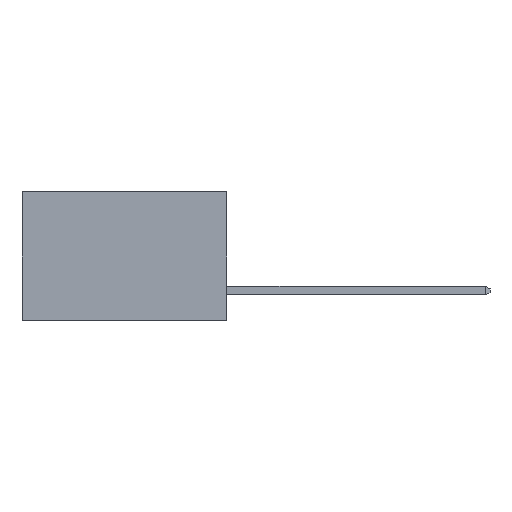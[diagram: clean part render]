
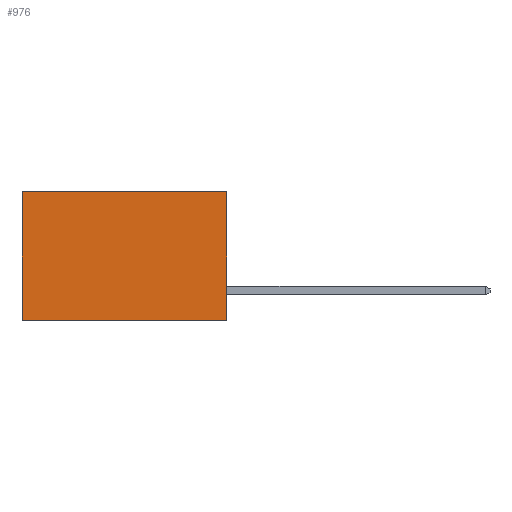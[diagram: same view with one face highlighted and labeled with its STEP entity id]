
A CAD part, left-side view. The second image highlights one B-rep face of the part: STEP entity #976.
In plain terms, the highlighted planar face has unit normal (-1, 0, 0).
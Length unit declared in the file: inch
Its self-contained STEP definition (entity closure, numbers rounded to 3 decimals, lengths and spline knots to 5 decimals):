
#465 = LINE ( 'NONE', #4557, #7526 ) ;
#525 = EDGE_CURVE ( 'NONE', #4774, #3673, #564, .T. ) ;
#564 = LINE ( 'NONE', #1978, #5940 ) ;
#807 = EDGE_CURVE ( 'NONE', #5442, #4774, #7591, .T. ) ;
#821 = CARTESIAN_POINT ( 'NONE',  ( 0.277, 0., -0.37 ) ) ;
#976 = ADVANCED_FACE ( 'NONE', ( #1510 ), #4227, .F. ) ;
#1510 = FACE_OUTER_BOUND ( 'NONE', #4595, .T. ) ;
#1978 = CARTESIAN_POINT ( 'NONE',  ( 0.277, 0., -0.37 ) ) ;
#2312 = DIRECTION ( 'NONE',  ( 0., 1., 0. ) ) ;
#2870 = AXIS2_PLACEMENT_3D ( 'NONE', #821, #4844, #5857 ) ;
#3120 = EDGE_CURVE ( 'NONE', #3223, #3673, #7224, .T. ) ;
#3223 = VERTEX_POINT ( 'NONE', #7795 ) ;
#3232 = CARTESIAN_POINT ( 'NONE',  ( 0.277, 0.59, -0.37 ) ) ;
#3463 = EDGE_CURVE ( 'NONE', #5442, #3223, #465, .T. ) ;
#3554 = VECTOR ( 'NONE', #3825, 39.37008 ) ;
#3673 = VERTEX_POINT ( 'NONE', #4017 ) ;
#3825 = DIRECTION ( 'NONE',  ( 0., 0., -1. ) ) ;
#4017 = CARTESIAN_POINT ( 'NONE',  ( 0.277, 0.59, -0.37 ) ) ;
#4227 = PLANE ( 'NONE',  #2870 ) ;
#4259 = DIRECTION ( 'NONE',  ( 0., 0., -1. ) ) ;
#4557 = CARTESIAN_POINT ( 'NONE',  ( 0.277, 0., 0. ) ) ;
#4595 = EDGE_LOOP ( 'NONE', ( #7276, #7112, #6226, #8085 ) ) ;
#4774 = VERTEX_POINT ( 'NONE', #7119 ) ;
#4778 = DIRECTION ( 'NONE',  ( 0., 1., 0. ) ) ;
#4844 = DIRECTION ( 'NONE',  ( 1., 0., 0. ) ) ;
#5442 = VERTEX_POINT ( 'NONE', #6352 ) ;
#5721 = VECTOR ( 'NONE', #4259, 39.37008 ) ;
#5857 = DIRECTION ( 'NONE',  ( 0., 0., -1. ) ) ;
#5940 = VECTOR ( 'NONE', #2312, 39.37008 ) ;
#6226 = ORIENTED_EDGE ( 'NONE', *, *, #807, .F. ) ;
#6352 = CARTESIAN_POINT ( 'NONE',  ( 0.277, 0., 0. ) ) ;
#7112 = ORIENTED_EDGE ( 'NONE', *, *, #525, .F. ) ;
#7119 = CARTESIAN_POINT ( 'NONE',  ( 0.277, 0., -0.37 ) ) ;
#7224 = LINE ( 'NONE', #3232, #3554 ) ;
#7276 = ORIENTED_EDGE ( 'NONE', *, *, #3120, .T. ) ;
#7330 = CARTESIAN_POINT ( 'NONE',  ( 0.277, 0., -0.37 ) ) ;
#7526 = VECTOR ( 'NONE', #4778, 39.37008 ) ;
#7591 = LINE ( 'NONE', #7330, #5721 ) ;
#7795 = CARTESIAN_POINT ( 'NONE',  ( 0.277, 0.59, 0. ) ) ;
#8085 = ORIENTED_EDGE ( 'NONE', *, *, #3463, .T. ) ;
